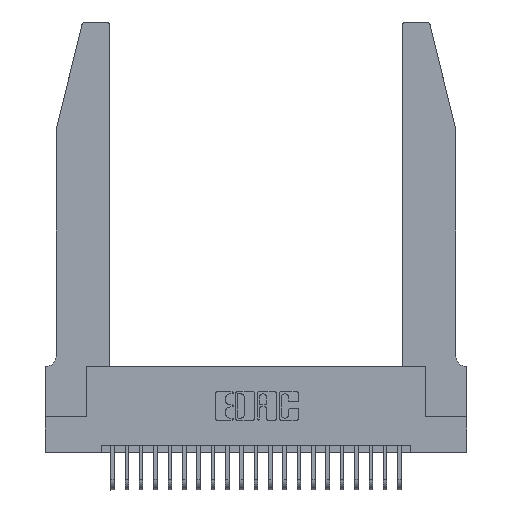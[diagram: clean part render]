
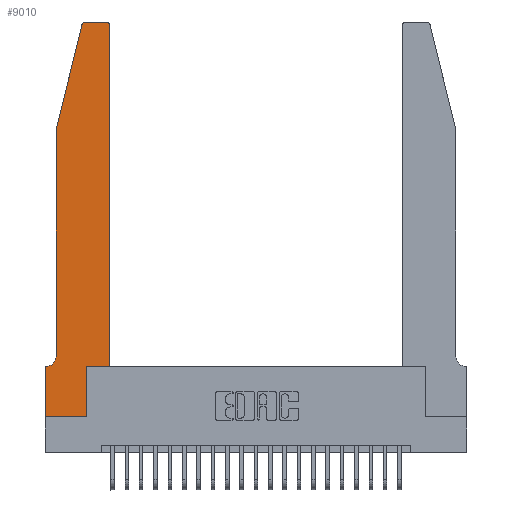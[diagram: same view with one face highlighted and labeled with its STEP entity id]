
A CAD part, top view. The second image highlights one B-rep face of the part: STEP entity #9010.
In plain terms, the highlighted planar face has unit normal (0, 0, 1).
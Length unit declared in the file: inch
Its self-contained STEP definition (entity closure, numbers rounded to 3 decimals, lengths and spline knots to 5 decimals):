
#52 = ORIENTED_EDGE ( 'NONE', *, *, #22507, .T. ) ;
#184 = CARTESIAN_POINT ( 'NONE',  ( 0.0755, 0.35, 0.37 ) ) ;
#185 = VERTEX_POINT ( 'NONE', #18436 ) ;
#294 = EDGE_CURVE ( 'NONE', #9666, #18569, #808, .T. ) ;
#429 = CARTESIAN_POINT ( 'NONE',  ( 0.4505, 2.72, 0.37 ) ) ;
#808 = CIRCLE ( 'NONE', #14016, 0.03 ) ;
#1308 = EDGE_CURVE ( 'NONE', #21047, #7511, #9814, .T. ) ;
#1406 = CARTESIAN_POINT ( 'NONE',  ( 0.2605, 2.75, 0.37 ) ) ;
#1423 = CARTESIAN_POINT ( 'NONE',  ( 0.4205, 2.75, 0.37 ) ) ;
#1450 = CARTESIAN_POINT ( 'NONE',  ( 0.0755, 0.42, 0.37 ) ) ;
#1736 = VECTOR ( 'NONE', #20889, 39.37008 ) ;
#1787 = CARTESIAN_POINT ( 'NONE',  ( 0., 0.35, 0.37 ) ) ;
#1852 = LINE ( 'NONE', #19364, #11089 ) ;
#2024 = VERTEX_POINT ( 'NONE', #429 ) ;
#2579 = DIRECTION ( 'NONE',  ( 0., 0., -1. ) ) ;
#3171 = VECTOR ( 'NONE', #7142, 39.37008 ) ;
#3419 = EDGE_CURVE ( 'NONE', #17706, #9666, #14716, .T. ) ;
#3422 = CARTESIAN_POINT ( 'NONE',  ( 0., 0., 0.37 ) ) ;
#3430 = CARTESIAN_POINT ( 'NONE',  ( 0.2865, 0., 0.37 ) ) ;
#3449 = DIRECTION ( 'NONE',  ( 0., -1., 0. ) ) ;
#3549 = VECTOR ( 'NONE', #3449, 39.37008 ) ;
#3644 = CARTESIAN_POINT ( 'NONE',  ( 0.0755, 2., 0.37 ) ) ;
#3688 = CARTESIAN_POINT ( 'NONE',  ( 0.4505, 0.35, 0.37 ) ) ;
#3820 = ORIENTED_EDGE ( 'NONE', *, *, #18181, .T. ) ;
#4251 = ORIENTED_EDGE ( 'NONE', *, *, #294, .T. ) ;
#4317 = AXIS2_PLACEMENT_3D ( 'NONE', #18618, #7816, #20426 ) ;
#4737 = EDGE_CURVE ( 'NONE', #2024, #17706, #15228, .T. ) ;
#5132 = EDGE_CURVE ( 'NONE', #185, #22950, #12666, .T. ) ;
#5349 = DIRECTION ( 'NONE',  ( 0., -1., 0. ) ) ;
#5542 = DIRECTION ( 'NONE',  ( 1., 0., 0. ) ) ;
#5802 = DIRECTION ( 'NONE',  ( -1., 0., 0. ) ) ;
#6019 = DIRECTION ( 'NONE',  ( -0.239, -0.971, 0. ) ) ;
#7142 = DIRECTION ( 'NONE',  ( 1., 0., 0. ) ) ;
#7341 = LINE ( 'NONE', #9866, #12172 ) ;
#7388 = EDGE_CURVE ( 'NONE', #11605, #2024, #1852, .T. ) ;
#7511 = VERTEX_POINT ( 'NONE', #1450 ) ;
#7683 = ORIENTED_EDGE ( 'NONE', *, *, #1308, .T. ) ;
#7816 = DIRECTION ( 'NONE',  ( 0., 0., 1. ) ) ;
#7863 = VECTOR ( 'NONE', #5802, 39.37008 ) ;
#8145 = FACE_OUTER_BOUND ( 'NONE', #15269, .T. ) ;
#8231 = EDGE_CURVE ( 'NONE', #22950, #10897, #8489, .T. ) ;
#8488 = CARTESIAN_POINT ( 'NONE',  ( 0.0755, 2., 0.37 ) ) ;
#8489 = LINE ( 'NONE', #14294, #3549 ) ;
#9010 = ADVANCED_FACE ( 'NONE', ( #8145 ), #12765, .T. ) ;
#9100 = CARTESIAN_POINT ( 'NONE',  ( 0., 0.35, 0.37 ) ) ;
#9236 = AXIS2_PLACEMENT_3D ( 'NONE', #13541, #2579, #15337 ) ;
#9666 = VERTEX_POINT ( 'NONE', #22224 ) ;
#9700 = ORIENTED_EDGE ( 'NONE', *, *, #10415, .T. ) ;
#9814 = LINE ( 'NONE', #3644, #23472 ) ;
#9866 = CARTESIAN_POINT ( 'NONE',  ( 0.4505, 0.35, 0.37 ) ) ;
#10175 = ORIENTED_EDGE ( 'NONE', *, *, #12458, .T. ) ;
#10415 = EDGE_CURVE ( 'NONE', #10897, #20082, #13476, .T. ) ;
#10897 = VERTEX_POINT ( 'NONE', #14164 ) ;
#10971 = ORIENTED_EDGE ( 'NONE', *, *, #19248, .T. ) ;
#11088 = VERTEX_POINT ( 'NONE', #20121 ) ;
#11089 = VECTOR ( 'NONE', #21166, 39.37008 ) ;
#11190 = DIRECTION ( 'NONE',  ( 1., 0., 0. ) ) ;
#11370 = DIRECTION ( 'NONE',  ( 0., 0., 1. ) ) ;
#11447 = CARTESIAN_POINT ( 'NONE',  ( 0.284, 2.72, 0.37 ) ) ;
#11605 = VERTEX_POINT ( 'NONE', #3688 ) ;
#11719 = VECTOR ( 'NONE', #6019, 39.37008 ) ;
#12172 = VECTOR ( 'NONE', #22362, 39.37008 ) ;
#12399 = DIRECTION ( 'NONE',  ( -1., 0., 0. ) ) ;
#12458 = EDGE_CURVE ( 'NONE', #18569, #21047, #21261, .T. ) ;
#12666 = LINE ( 'NONE', #184, #7863 ) ;
#12765 = PLANE ( 'NONE',  #17141 ) ;
#13054 = ORIENTED_EDGE ( 'NONE', *, *, #4737, .T. ) ;
#13476 = LINE ( 'NONE', #3422, #3171 ) ;
#13541 = CARTESIAN_POINT ( 'NONE',  ( 0.0055, 0.42, 0.37 ) ) ;
#13660 = CARTESIAN_POINT ( 'NONE',  ( 0.2865, 0.35, 0.37 ) ) ;
#14016 = AXIS2_PLACEMENT_3D ( 'NONE', #11447, #11370, #11190 ) ;
#14164 = CARTESIAN_POINT ( 'NONE',  ( 0., 0., 0.37 ) ) ;
#14294 = CARTESIAN_POINT ( 'NONE',  ( 0., 0., 0.37 ) ) ;
#14716 = LINE ( 'NONE', #1406, #18950 ) ;
#15228 = CIRCLE ( 'NONE', #4317, 0.03 ) ;
#15269 = EDGE_LOOP ( 'NONE', ( #16620, #4251, #10175, #7683, #10971, #18786, #15635, #9700, #3820, #52, #18455, #13054 ) ) ;
#15337 = DIRECTION ( 'NONE',  ( -1., 0., 0. ) ) ;
#15635 = ORIENTED_EDGE ( 'NONE', *, *, #8231, .T. ) ;
#16379 = DIRECTION ( 'NONE',  ( 0., 0., 1. ) ) ;
#16620 = ORIENTED_EDGE ( 'NONE', *, *, #3419, .T. ) ;
#17141 = AXIS2_PLACEMENT_3D ( 'NONE', #1787, #16379, #5542 ) ;
#17706 = VERTEX_POINT ( 'NONE', #1423 ) ;
#18181 = EDGE_CURVE ( 'NONE', #20082, #11088, #23279, .T. ) ;
#18436 = CARTESIAN_POINT ( 'NONE',  ( 0.0055, 0.35, 0.37 ) ) ;
#18455 = ORIENTED_EDGE ( 'NONE', *, *, #7388, .T. ) ;
#18569 = VERTEX_POINT ( 'NONE', #20730 ) ;
#18618 = CARTESIAN_POINT ( 'NONE',  ( 0.4205, 2.72, 0.37 ) ) ;
#18671 = CARTESIAN_POINT ( 'NONE',  ( 0.0755, 2., 0.37 ) ) ;
#18786 = ORIENTED_EDGE ( 'NONE', *, *, #5132, .T. ) ;
#18950 = VECTOR ( 'NONE', #12399, 39.37008 ) ;
#19248 = EDGE_CURVE ( 'NONE', #7511, #185, #22662, .T. ) ;
#19364 = CARTESIAN_POINT ( 'NONE',  ( 0.4505, 0.35, 0.37 ) ) ;
#20082 = VERTEX_POINT ( 'NONE', #3430 ) ;
#20121 = CARTESIAN_POINT ( 'NONE',  ( 0.2865, 0.35, 0.37 ) ) ;
#20426 = DIRECTION ( 'NONE',  ( 1., 0., 0. ) ) ;
#20730 = CARTESIAN_POINT ( 'NONE',  ( 0.25487, 2.72718, 0.37 ) ) ;
#20889 = DIRECTION ( 'NONE',  ( 0., 1., 0. ) ) ;
#21047 = VERTEX_POINT ( 'NONE', #8488 ) ;
#21166 = DIRECTION ( 'NONE',  ( 0., 1., 0. ) ) ;
#21261 = LINE ( 'NONE', #18671, #11719 ) ;
#22224 = CARTESIAN_POINT ( 'NONE',  ( 0.284, 2.75, 0.37 ) ) ;
#22362 = DIRECTION ( 'NONE',  ( 1., 0., 0. ) ) ;
#22507 = EDGE_CURVE ( 'NONE', #11088, #11605, #7341, .T. ) ;
#22662 = CIRCLE ( 'NONE', #9236, 0.07 ) ;
#22950 = VERTEX_POINT ( 'NONE', #9100 ) ;
#23279 = LINE ( 'NONE', #13660, #1736 ) ;
#23472 = VECTOR ( 'NONE', #5349, 39.37008 ) ;
